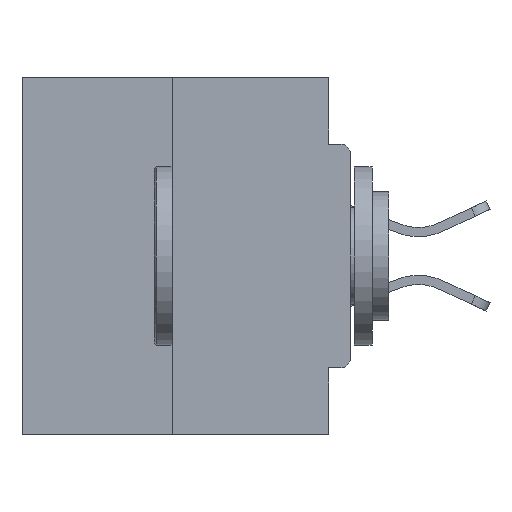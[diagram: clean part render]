
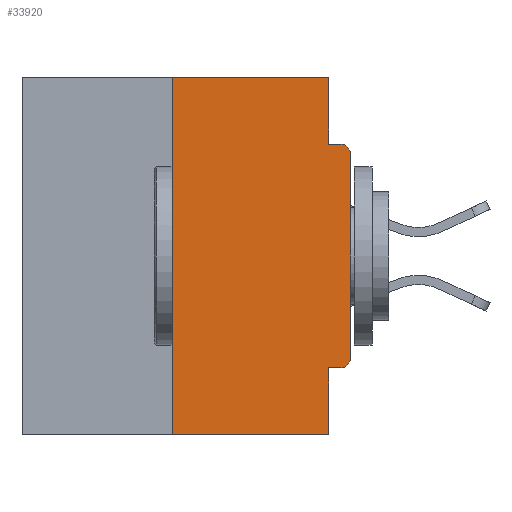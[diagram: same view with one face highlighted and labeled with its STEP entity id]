
A CAD part, left-side view. The second image highlights one B-rep face of the part: STEP entity #33920.
In plain terms, the highlighted planar face has unit normal (-1, 0, 0).
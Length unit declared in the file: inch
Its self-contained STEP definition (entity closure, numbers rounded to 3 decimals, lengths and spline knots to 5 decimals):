
#271 = EDGE_CURVE ( 'NONE', #26950, #11915, #38465, .T. ) ;
#477 = ORIENTED_EDGE ( 'NONE', *, *, #28092, .F. ) ;
#728 = ORIENTED_EDGE ( 'NONE', *, *, #271, .T. ) ;
#3298 = DIRECTION ( 'NONE',  ( 0., 0., -1. ) ) ;
#3415 = AXIS2_PLACEMENT_3D ( 'NONE', #43350, #10369, #32164 ) ;
#3761 = CARTESIAN_POINT ( 'NONE',  ( 0., 0.015, -0.0935 ) ) ;
#3966 = LINE ( 'NONE', #24074, #44906 ) ;
#4810 = DIRECTION ( 'NONE',  ( 0., 1., 0. ) ) ;
#4911 = AXIS2_PLACEMENT_3D ( 'NONE', #16697, #34938, #12408 ) ;
#4941 = ORIENTED_EDGE ( 'NONE', *, *, #30270, .T. ) ;
#5329 = CARTESIAN_POINT ( 'NONE',  ( 0., 0.25, -0.5 ) ) ;
#5492 = CARTESIAN_POINT ( 'NONE',  ( 0., 0.25, 0. ) ) ;
#5848 = VERTEX_POINT ( 'NONE', #28831 ) ;
#6299 = PLANE ( 'NONE',  #3415 ) ;
#8721 = EDGE_LOOP ( 'NONE', ( #11502, #36574, #728, #21150, #33839, #4941, #41257, #36792, #477, #34371 ) ) ;
#9086 = CARTESIAN_POINT ( 'NONE',  ( 0., 0.031, 0. ) ) ;
#9107 = CARTESIAN_POINT ( 'NONE',  ( 0., 0.031, 0. ) ) ;
#9189 = EDGE_CURVE ( 'NONE', #24486, #11915, #39285, .T. ) ;
#9225 = FACE_OUTER_BOUND ( 'NONE', #8721, .T. ) ;
#9761 = EDGE_CURVE ( 'NONE', #5848, #24486, #28855, .T. ) ;
#10369 = DIRECTION ( 'NONE',  ( 1., 0., 0. ) ) ;
#10891 = EDGE_CURVE ( 'NONE', #24940, #12972, #26465, .T. ) ;
#11502 = ORIENTED_EDGE ( 'NONE', *, *, #13841, .F. ) ;
#11880 = DIRECTION ( 'NONE',  ( -1., 0., 0. ) ) ;
#11915 = VERTEX_POINT ( 'NONE', #44261 ) ;
#12408 = DIRECTION ( 'NONE',  ( 0., 0., -1. ) ) ;
#12972 = VERTEX_POINT ( 'NONE', #34051 ) ;
#13258 = DIRECTION ( 'NONE',  ( 0., 0., 1. ) ) ;
#13460 = LINE ( 'NONE', #47122, #37094 ) ;
#13683 = CARTESIAN_POINT ( 'NONE',  ( 0., 0.031, -0.5 ) ) ;
#13841 = EDGE_CURVE ( 'NONE', #47290, #24940, #20654, .T. ) ;
#15744 = AXIS2_PLACEMENT_3D ( 'NONE', #38123, #11880, #30890 ) ;
#16037 = CARTESIAN_POINT ( 'NONE',  ( 0., 0., -0.1085 ) ) ;
#16656 = EDGE_CURVE ( 'NONE', #26950, #47290, #19231, .T. ) ;
#16697 = CARTESIAN_POINT ( 'NONE',  ( 0., 0.015, -0.1085 ) ) ;
#19231 = LINE ( 'NONE', #21372, #20972 ) ;
#19287 = EDGE_CURVE ( 'NONE', #40413, #29561, #3966, .T. ) ;
#20654 = LINE ( 'NONE', #29382, #31060 ) ;
#20972 = VECTOR ( 'NONE', #47059, 39.37008 ) ;
#21150 = ORIENTED_EDGE ( 'NONE', *, *, #9189, .F. ) ;
#21372 = CARTESIAN_POINT ( 'NONE',  ( 0., 0.25, 0. ) ) ;
#22141 = DIRECTION ( 'NONE',  ( 0., -1., 0. ) ) ;
#22549 = VECTOR ( 'NONE', #3298, 39.37008 ) ;
#24074 = CARTESIAN_POINT ( 'NONE',  ( 0., 0., 0. ) ) ;
#24486 = VERTEX_POINT ( 'NONE', #29316 ) ;
#24940 = VERTEX_POINT ( 'NONE', #9107 ) ;
#25102 = DIRECTION ( 'NONE',  ( 0., -1., 0. ) ) ;
#26465 = LINE ( 'NONE', #9086, #35646 ) ;
#26950 = VERTEX_POINT ( 'NONE', #5329 ) ;
#28092 = EDGE_CURVE ( 'NONE', #12972, #47705, #13460, .T. ) ;
#28652 = VECTOR ( 'NONE', #22141, 39.37008 ) ;
#28831 = CARTESIAN_POINT ( 'NONE',  ( 0., 0.015, -0.4065 ) ) ;
#28855 = LINE ( 'NONE', #45073, #47237 ) ;
#28889 = DIRECTION ( 'NONE',  ( 0., -1., 0. ) ) ;
#29316 = CARTESIAN_POINT ( 'NONE',  ( 0., 0.031, -0.4065 ) ) ;
#29382 = CARTESIAN_POINT ( 'NONE',  ( 0., 0.46, 0. ) ) ;
#29561 = VERTEX_POINT ( 'NONE', #16037 ) ;
#29802 = CIRCLE ( 'NONE', #4911, 0.015 ) ;
#30270 = EDGE_CURVE ( 'NONE', #5848, #40413, #39740, .T. ) ;
#30890 = DIRECTION ( 'NONE',  ( 0., 0., -1. ) ) ;
#31060 = VECTOR ( 'NONE', #28889, 39.37008 ) ;
#31348 = DIRECTION ( 'NONE',  ( 0., 0., -1. ) ) ;
#31820 = EDGE_CURVE ( 'NONE', #29561, #47705, #29802, .T. ) ;
#32164 = DIRECTION ( 'NONE',  ( 0., 0., -1. ) ) ;
#33525 = CARTESIAN_POINT ( 'NONE',  ( 0., 0., -0.3915 ) ) ;
#33839 = ORIENTED_EDGE ( 'NONE', *, *, #9761, .F. ) ;
#33920 = ADVANCED_FACE ( 'NONE', ( #9225 ), #6299, .F. ) ;
#34051 = CARTESIAN_POINT ( 'NONE',  ( 0., 0.031, -0.0935 ) ) ;
#34371 = ORIENTED_EDGE ( 'NONE', *, *, #10891, .F. ) ;
#34938 = DIRECTION ( 'NONE',  ( -1., 0., 0. ) ) ;
#35646 = VECTOR ( 'NONE', #31348, 39.37008 ) ;
#36574 = ORIENTED_EDGE ( 'NONE', *, *, #16656, .F. ) ;
#36792 = ORIENTED_EDGE ( 'NONE', *, *, #31820, .T. ) ;
#37094 = VECTOR ( 'NONE', #25102, 39.37008 ) ;
#38123 = CARTESIAN_POINT ( 'NONE',  ( 0., 0.015, -0.3915 ) ) ;
#38465 = LINE ( 'NONE', #40471, #28652 ) ;
#39285 = LINE ( 'NONE', #13683, #22549 ) ;
#39740 = CIRCLE ( 'NONE', #15744, 0.015 ) ;
#40413 = VERTEX_POINT ( 'NONE', #33525 ) ;
#40471 = CARTESIAN_POINT ( 'NONE',  ( 0., 0.46, -0.5 ) ) ;
#41257 = ORIENTED_EDGE ( 'NONE', *, *, #19287, .T. ) ;
#43350 = CARTESIAN_POINT ( 'NONE',  ( 0., 0.46, 0. ) ) ;
#44261 = CARTESIAN_POINT ( 'NONE',  ( 0., 0.031, -0.5 ) ) ;
#44906 = VECTOR ( 'NONE', #13258, 39.37008 ) ;
#45073 = CARTESIAN_POINT ( 'NONE',  ( 0., 0., -0.4065 ) ) ;
#47059 = DIRECTION ( 'NONE',  ( 0., 0., 1. ) ) ;
#47122 = CARTESIAN_POINT ( 'NONE',  ( 0., 0., -0.0935 ) ) ;
#47237 = VECTOR ( 'NONE', #4810, 39.37008 ) ;
#47290 = VERTEX_POINT ( 'NONE', #5492 ) ;
#47705 = VERTEX_POINT ( 'NONE', #3761 ) ;
